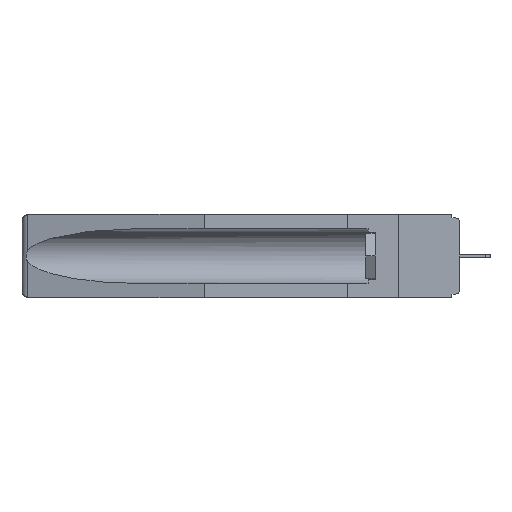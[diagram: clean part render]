
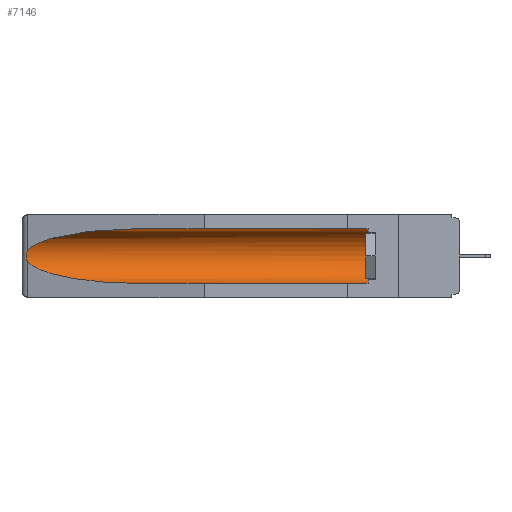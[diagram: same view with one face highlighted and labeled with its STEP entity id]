
A CAD part, left-side view. The second image highlights one B-rep face of the part: STEP entity #7146.
In plain terms, the highlighted cylindrical face has radius 2.857 mm (diameter 5.715 mm), a partial arc.
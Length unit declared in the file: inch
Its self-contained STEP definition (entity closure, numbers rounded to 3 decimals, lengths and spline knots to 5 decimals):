
#314 = ORIENTED_EDGE ( 'NONE', *, *, #12465, .T. ) ;
#982 =( BOUNDED_CURVE ( )  B_SPLINE_CURVE ( 3, ( #4259, #3016, #6875, #12026 ),
 .UNSPECIFIED., .F., .T. ) 
 B_SPLINE_CURVE_WITH_KNOTS ( ( 4, 4 ),
 ( 0.1948, 1.5708 ),
 .UNSPECIFIED. ) 
 CURVE ( )  GEOMETRIC_REPRESENTATION_ITEM ( )  RATIONAL_B_SPLINE_CURVE ( ( 1., 0.848, 0.848, 1. ) ) 
 REPRESENTATION_ITEM ( '' )  );
#1315 = CARTESIAN_POINT ( 'NONE',  ( 0.26537, 1.52718, -0.14972 ) ) ;
#1520 = DIRECTION ( 'NONE',  ( 0., 0., 1. ) ) ;
#1806 = CARTESIAN_POINT ( 'NONE',  ( 0.155, 1.07973, -0.059 ) ) ;
#1856 = ORIENTED_EDGE ( 'NONE', *, *, #12575, .T. ) ;
#2562 = CARTESIAN_POINT ( 'NONE',  ( 0.2673, 1.53269, -0.17917 ) ) ;
#3016 = CARTESIAN_POINT ( 'NONE',  ( 0.25451, 1.48313, -0.24835 ) ) ;
#3648 = CARTESIAN_POINT ( 'NONE',  ( 0.26597, 1.5296, -0.19026 ) ) ;
#3940 = CARTESIAN_POINT ( 'NONE',  ( 0.155, 1.07973, -0.284 ) ) ;
#4156 = ORIENTED_EDGE ( 'NONE', *, *, #6637, .F. ) ;
#4259 = CARTESIAN_POINT ( 'NONE',  ( 0.26537, 1.52718, -0.19328 ) ) ;
#4488 = AXIS2_PLACEMENT_3D ( 'NONE', #16504, #12673, #1520 ) ;
#4578 = EDGE_CURVE ( 'NONE', #13124, #5615, #982, .T. ) ;
#5149 = CARTESIAN_POINT ( 'NONE',  ( 0.26655, 1.53094, -0.18657 ) ) ;
#5443 = DIRECTION ( 'NONE',  ( 0., 1., 0. ) ) ;
#5615 = VERTEX_POINT ( 'NONE', #3940 ) ;
#6558 = CARTESIAN_POINT ( 'NONE',  ( 0.155, 1.07973, -0.059 ) ) ;
#6637 = EDGE_CURVE ( 'NONE', #7533, #5615, #8121, .T. ) ;
#6875 = CARTESIAN_POINT ( 'NONE',  ( 0.21114, 1.30732, -0.284 ) ) ;
#6900 = VERTEX_POINT ( 'NONE', #1806 ) ;
#6908 = VECTOR ( 'NONE', #5443, 39.37008 ) ;
#7146 = ADVANCED_FACE ( 'NONE', ( #11053 ), #12409, .F. ) ;
#7533 = VERTEX_POINT ( 'NONE', #15258 ) ;
#7895 = LINE ( 'NONE', #12902, #6908 ) ;
#8121 = LINE ( 'NONE', #10570, #13903 ) ;
#8389 = CARTESIAN_POINT ( 'NONE',  ( 0.26537, 1.52718, -0.19328 ) ) ;
#8677 = DIRECTION ( 'NONE',  ( 0., 0., 1. ) ) ;
#8765 = VERTEX_POINT ( 'NONE', #12300 ) ;
#9125 = CARTESIAN_POINT ( 'NONE',  ( 0.2673, 1.5327, -0.16383 ) ) ;
#9478 = DIRECTION ( 'NONE',  ( 0., 1., 0. ) ) ;
#9921 = CARTESIAN_POINT ( 'NONE',  ( 0.26537, 1.52718, -0.14972 ) ) ;
#10035 = EDGE_LOOP ( 'NONE', ( #11577, #16098, #15488, #4156, #314, #1856 ) ) ;
#10228 = CARTESIAN_POINT ( 'NONE',  ( 0.2675, 1.53308, -0.16763 ) ) ;
#10440 = CARTESIAN_POINT ( 'NONE',  ( 0.25451, 1.48313, -0.09465 ) ) ;
#10570 = CARTESIAN_POINT ( 'NONE',  ( 0.155, -0.30754, -0.284 ) ) ;
#11053 = FACE_OUTER_BOUND ( 'NONE', #10035, .T. ) ;
#11164 = B_SPLINE_CURVE_WITH_KNOTS ( 'NONE', 3,
 ( #1315, #15483, #14125, #9125, #10228, #15403, #2562, #5149, #3648, #13965 ),
 .UNSPECIFIED., .F., .F.,
 ( 4, 2, 2, 2, 4 ),
 ( 0., 0.00029, 0.00058, 0.00087, 0.00117 ),
 .UNSPECIFIED. ) ;
#11519 = VERTEX_POINT ( 'NONE', #9921 ) ;
#11577 = ORIENTED_EDGE ( 'NONE', *, *, #15464, .T. ) ;
#11793 = CARTESIAN_POINT ( 'NONE',  ( 0.26537, 1.52718, -0.14972 ) ) ;
#12026 = CARTESIAN_POINT ( 'NONE',  ( 0.155, 1.07973, -0.284 ) ) ;
#12300 = CARTESIAN_POINT ( 'NONE',  ( 0.155, 0.126, -0.059 ) ) ;
#12409 = CYLINDRICAL_SURFACE ( 'NONE', #4488, 0.1125 ) ;
#12465 = EDGE_CURVE ( 'NONE', #7533, #8765, #12585, .T. ) ;
#12575 = EDGE_CURVE ( 'NONE', #8765, #6900, #7895, .T. ) ;
#12585 = CIRCLE ( 'NONE', #15304, 0.1125 ) ;
#12673 = DIRECTION ( 'NONE',  ( 0., 1., 0. ) ) ;
#12902 = CARTESIAN_POINT ( 'NONE',  ( 0.155, -0.30754, -0.059 ) ) ;
#13074 = CARTESIAN_POINT ( 'NONE',  ( 0.21114, 1.30732, -0.059 ) ) ;
#13124 = VERTEX_POINT ( 'NONE', #8389 ) ;
#13903 = VECTOR ( 'NONE', #9478, 39.37008 ) ;
#13935 =( BOUNDED_CURVE ( )  B_SPLINE_CURVE ( 3, ( #6558, #13074, #10440, #11793 ),
 .UNSPECIFIED., .F., .T. ) 
 B_SPLINE_CURVE_WITH_KNOTS ( ( 4, 4 ),
 ( 4.71239, 6.08839 ),
 .UNSPECIFIED. ) 
 CURVE ( )  GEOMETRIC_REPRESENTATION_ITEM ( )  RATIONAL_B_SPLINE_CURVE ( ( 1., 0.848, 0.848, 1. ) ) 
 REPRESENTATION_ITEM ( '' )  );
#13965 = CARTESIAN_POINT ( 'NONE',  ( 0.26537, 1.52718, -0.19328 ) ) ;
#14125 = CARTESIAN_POINT ( 'NONE',  ( 0.26654, 1.53092, -0.15636 ) ) ;
#15131 = CARTESIAN_POINT ( 'NONE',  ( 0.155, 0.126, -0.1715 ) ) ;
#15258 = CARTESIAN_POINT ( 'NONE',  ( 0.155, 0.126, -0.284 ) ) ;
#15304 = AXIS2_PLACEMENT_3D ( 'NONE', #15131, #16645, #8677 ) ;
#15403 = CARTESIAN_POINT ( 'NONE',  ( 0.2675, 1.53308, -0.17534 ) ) ;
#15464 = EDGE_CURVE ( 'NONE', #6900, #11519, #13935, .T. ) ;
#15483 = CARTESIAN_POINT ( 'NONE',  ( 0.26597, 1.52961, -0.15275 ) ) ;
#15488 = ORIENTED_EDGE ( 'NONE', *, *, #4578, .T. ) ;
#16057 = EDGE_CURVE ( 'NONE', #11519, #13124, #11164, .T. ) ;
#16098 = ORIENTED_EDGE ( 'NONE', *, *, #16057, .T. ) ;
#16504 = CARTESIAN_POINT ( 'NONE',  ( 0.155, -0.30754, -0.1715 ) ) ;
#16645 = DIRECTION ( 'NONE',  ( 0., -1., 0. ) ) ;
